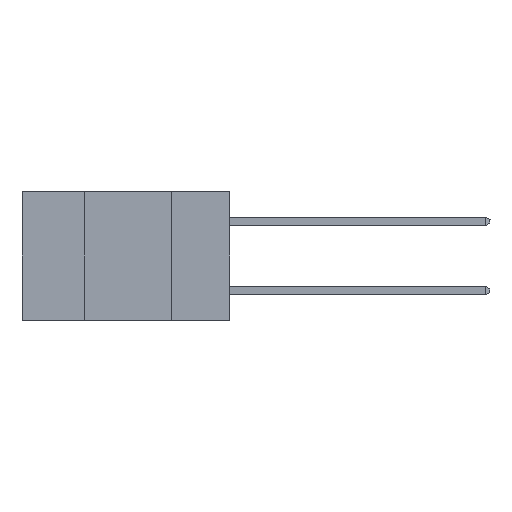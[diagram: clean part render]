
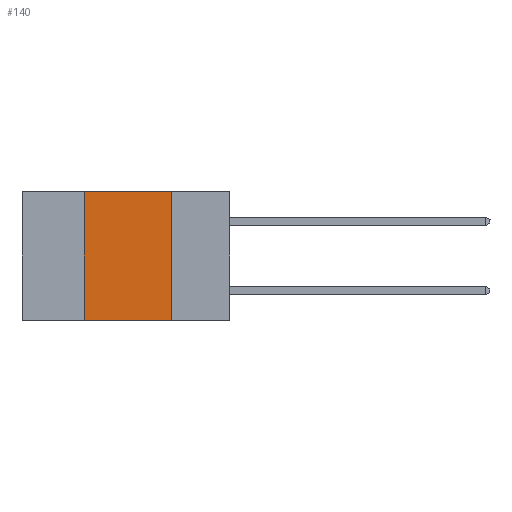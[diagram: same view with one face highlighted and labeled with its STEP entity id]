
A CAD part, left-side view. The second image highlights one B-rep face of the part: STEP entity #140.
In plain terms, the highlighted planar face has unit normal (-1, 0, 0).
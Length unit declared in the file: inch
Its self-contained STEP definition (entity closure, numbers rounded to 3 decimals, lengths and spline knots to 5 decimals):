
#140 = ADVANCED_FACE ( 'NONE', ( #3760 ), #10022, .F. ) ;
#150 = VECTOR ( 'NONE', #16250, 39.37008 ) ;
#1145 = VERTEX_POINT ( 'NONE', #7224 ) ;
#2206 = VERTEX_POINT ( 'NONE', #18578 ) ;
#2326 = ORIENTED_EDGE ( 'NONE', *, *, #16616, .T. ) ;
#2451 = CARTESIAN_POINT ( 'NONE',  ( 0., 0.42, -0.37 ) ) ;
#2780 = ORIENTED_EDGE ( 'NONE', *, *, #16160, .F. ) ;
#3760 = FACE_OUTER_BOUND ( 'NONE', #4385, .T. ) ;
#4142 = DIRECTION ( 'NONE',  ( 0., 0., 1. ) ) ;
#4151 = DIRECTION ( 'NONE',  ( 0., 0., -1. ) ) ;
#4385 = EDGE_LOOP ( 'NONE', ( #11160, #8027, #2780, #2326 ) ) ;
#5335 = EDGE_CURVE ( 'NONE', #1145, #17719, #9187, .T. ) ;
#5387 = AXIS2_PLACEMENT_3D ( 'NONE', #17782, #15887, #4151 ) ;
#5449 = LINE ( 'NONE', #17572, #17028 ) ;
#5932 = VERTEX_POINT ( 'NONE', #17010 ) ;
#6542 = EDGE_CURVE ( 'NONE', #17719, #5932, #5449, .T. ) ;
#7120 = LINE ( 'NONE', #2451, #12207 ) ;
#7224 = CARTESIAN_POINT ( 'NONE',  ( 0., 0.42, 0. ) ) ;
#7293 = CARTESIAN_POINT ( 'NONE',  ( 0., 0.17, 0. ) ) ;
#7455 = VECTOR ( 'NONE', #9091, 39.37008 ) ;
#8027 = ORIENTED_EDGE ( 'NONE', *, *, #5335, .F. ) ;
#9091 = DIRECTION ( 'NONE',  ( 0., -1., 0. ) ) ;
#9187 = LINE ( 'NONE', #12367, #7455 ) ;
#10022 = PLANE ( 'NONE',  #5387 ) ;
#11160 = ORIENTED_EDGE ( 'NONE', *, *, #6542, .F. ) ;
#11610 = DIRECTION ( 'NONE',  ( 0., 0., -1. ) ) ;
#12207 = VECTOR ( 'NONE', #4142, 39.37008 ) ;
#12367 = CARTESIAN_POINT ( 'NONE',  ( 0., 0.6, 0. ) ) ;
#15887 = DIRECTION ( 'NONE',  ( 1., 0., 0. ) ) ;
#16160 = EDGE_CURVE ( 'NONE', #2206, #1145, #7120, .T. ) ;
#16250 = DIRECTION ( 'NONE',  ( 0., -1., 0. ) ) ;
#16616 = EDGE_CURVE ( 'NONE', #2206, #5932, #18845, .T. ) ;
#17010 = CARTESIAN_POINT ( 'NONE',  ( 0., 0.17, -0.37 ) ) ;
#17028 = VECTOR ( 'NONE', #11610, 39.37008 ) ;
#17572 = CARTESIAN_POINT ( 'NONE',  ( 0., 0.17, -0.37 ) ) ;
#17719 = VERTEX_POINT ( 'NONE', #7293 ) ;
#17782 = CARTESIAN_POINT ( 'NONE',  ( 0., 0.6, 0. ) ) ;
#18578 = CARTESIAN_POINT ( 'NONE',  ( 0., 0.42, -0.37 ) ) ;
#18845 = LINE ( 'NONE', #19148, #150 ) ;
#19148 = CARTESIAN_POINT ( 'NONE',  ( 0., 0.6, -0.37 ) ) ;
